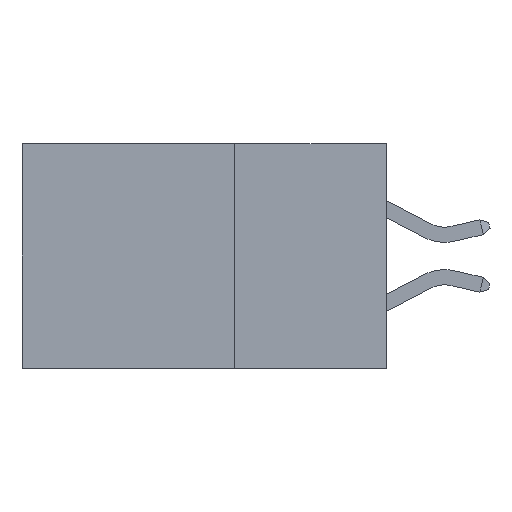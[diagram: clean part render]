
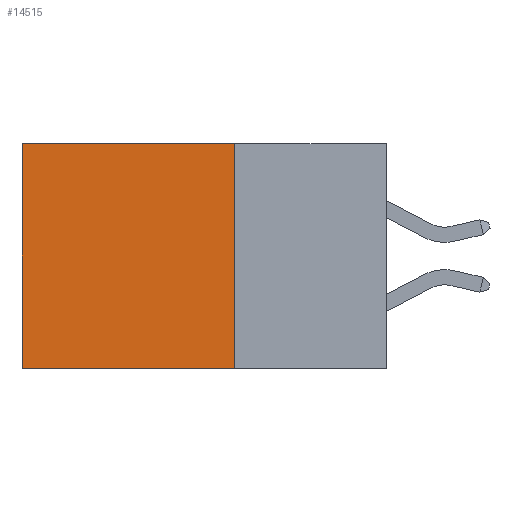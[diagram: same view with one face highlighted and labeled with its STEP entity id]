
A CAD part, left-side view. The second image highlights one B-rep face of the part: STEP entity #14515.
In plain terms, the highlighted planar face has unit normal (-1, 0, 0).
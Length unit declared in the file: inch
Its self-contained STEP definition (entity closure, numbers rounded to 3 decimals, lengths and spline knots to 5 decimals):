
#184 = DIRECTION ( 'NONE',  ( 0., 0., -1. ) ) ;
#2307 = VERTEX_POINT ( 'NONE', #4912 ) ;
#2337 = CARTESIAN_POINT ( 'NONE',  ( 0.298, 0.6, 0. ) ) ;
#2591 = FACE_OUTER_BOUND ( 'NONE', #17443, .T. ) ;
#2875 = LINE ( 'NONE', #2337, #8924 ) ;
#3982 = DIRECTION ( 'NONE',  ( 0., 1., 0. ) ) ;
#4808 = LINE ( 'NONE', #10972, #18293 ) ;
#4912 = CARTESIAN_POINT ( 'NONE',  ( 0.298, 0.6, -0.37 ) ) ;
#5241 = VERTEX_POINT ( 'NONE', #12204 ) ;
#5585 = CARTESIAN_POINT ( 'NONE',  ( 0.298, 0.25, 0. ) ) ;
#6245 = EDGE_CURVE ( 'NONE', #7897, #2307, #21199, .T. ) ;
#6621 = EDGE_CURVE ( 'NONE', #5241, #2307, #2875, .T. ) ;
#7897 = VERTEX_POINT ( 'NONE', #13527 ) ;
#8044 = DIRECTION ( 'NONE',  ( 0., 0., -1. ) ) ;
#8236 = ORIENTED_EDGE ( 'NONE', *, *, #6621, .T. ) ;
#8924 = VECTOR ( 'NONE', #8044, 39.37008 ) ;
#10280 = EDGE_CURVE ( 'NONE', #10508, #7897, #4808, .T. ) ;
#10508 = VERTEX_POINT ( 'NONE', #5585 ) ;
#10972 = CARTESIAN_POINT ( 'NONE',  ( 0.298, 0.25, 0. ) ) ;
#11168 = VECTOR ( 'NONE', #21170, 39.37008 ) ;
#12204 = CARTESIAN_POINT ( 'NONE',  ( 0.298, 0.6, 0. ) ) ;
#13190 = CARTESIAN_POINT ( 'NONE',  ( 0.298, 0.25, 0. ) ) ;
#13527 = CARTESIAN_POINT ( 'NONE',  ( 0.298, 0.25, -0.37 ) ) ;
#14508 = AXIS2_PLACEMENT_3D ( 'NONE', #13190, #16768, #20440 ) ;
#14515 = ADVANCED_FACE ( 'NONE', ( #2591 ), #20372, .F. ) ;
#15650 = CARTESIAN_POINT ( 'NONE',  ( 0.298, 0.25, 0. ) ) ;
#16587 = LINE ( 'NONE', #15650, #11168 ) ;
#16768 = DIRECTION ( 'NONE',  ( 1., 0., 0. ) ) ;
#17264 = ORIENTED_EDGE ( 'NONE', *, *, #18953, .T. ) ;
#17443 = EDGE_LOOP ( 'NONE', ( #8236, #21661, #18779, #17264 ) ) ;
#18293 = VECTOR ( 'NONE', #184, 39.37008 ) ;
#18555 = CARTESIAN_POINT ( 'NONE',  ( 0.298, 0.25, -0.37 ) ) ;
#18779 = ORIENTED_EDGE ( 'NONE', *, *, #10280, .F. ) ;
#18953 = EDGE_CURVE ( 'NONE', #10508, #5241, #16587, .T. ) ;
#20372 = PLANE ( 'NONE',  #14508 ) ;
#20440 = DIRECTION ( 'NONE',  ( 0., 0., -1. ) ) ;
#21170 = DIRECTION ( 'NONE',  ( 0., 1., 0. ) ) ;
#21199 = LINE ( 'NONE', #18555, #21504 ) ;
#21504 = VECTOR ( 'NONE', #3982, 39.37008 ) ;
#21661 = ORIENTED_EDGE ( 'NONE', *, *, #6245, .F. ) ;
